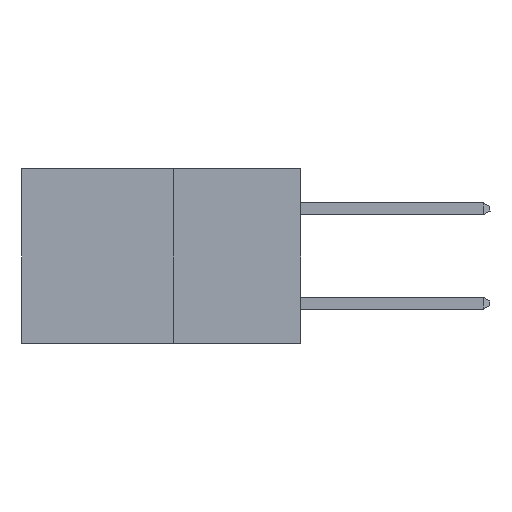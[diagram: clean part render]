
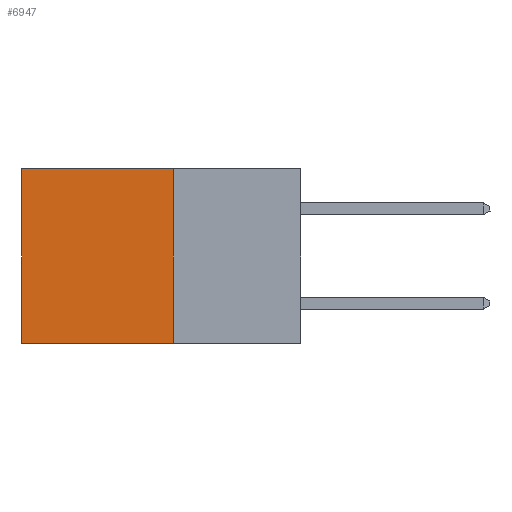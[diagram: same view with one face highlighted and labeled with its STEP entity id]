
A CAD part, left-side view. The second image highlights one B-rep face of the part: STEP entity #6947.
In plain terms, the highlighted planar face has unit normal (-1, 0, 0).
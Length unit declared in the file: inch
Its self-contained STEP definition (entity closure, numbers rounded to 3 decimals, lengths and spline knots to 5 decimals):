
#608 = VERTEX_POINT ( 'NONE', #18790 ) ;
#824 = LINE ( 'NONE', #18918, #17381 ) ;
#1024 = LINE ( 'NONE', #18147, #11940 ) ;
#1056 = CARTESIAN_POINT ( 'NONE',  ( 0.277, 0.27, -0.37 ) ) ;
#1272 = ORIENTED_EDGE ( 'NONE', *, *, #23942, .F. ) ;
#1971 = EDGE_LOOP ( 'NONE', ( #13141, #4662, #1272, #6593 ) ) ;
#3967 = DIRECTION ( 'NONE',  ( 0., 0., -1. ) ) ;
#4662 = ORIENTED_EDGE ( 'NONE', *, *, #21241, .F. ) ;
#6593 = ORIENTED_EDGE ( 'NONE', *, *, #24216, .T. ) ;
#6947 = ADVANCED_FACE ( 'NONE', ( #19543 ), #9834, .F. ) ;
#7674 = VECTOR ( 'NONE', #22424, 39.37008 ) ;
#8910 = AXIS2_PLACEMENT_3D ( 'NONE', #12114, #12168, #12165 ) ;
#9090 = CARTESIAN_POINT ( 'NONE',  ( 0.277, 0.27, 0. ) ) ;
#9834 = PLANE ( 'NONE',  #8910 ) ;
#11188 = CARTESIAN_POINT ( 'NONE',  ( 0.277, 0.59, -0.37 ) ) ;
#11940 = VECTOR ( 'NONE', #20237, 39.37008 ) ;
#12114 = CARTESIAN_POINT ( 'NONE',  ( 0.277, 0.27, -0.37 ) ) ;
#12165 = DIRECTION ( 'NONE',  ( 0., 0., -1. ) ) ;
#12168 = DIRECTION ( 'NONE',  ( 1., 0., 0. ) ) ;
#13141 = ORIENTED_EDGE ( 'NONE', *, *, #23037, .T. ) ;
#13915 = CARTESIAN_POINT ( 'NONE',  ( 0.277, 0.59, 0. ) ) ;
#15247 = CARTESIAN_POINT ( 'NONE',  ( 0.277, 0.27, 0. ) ) ;
#15305 = VERTEX_POINT ( 'NONE', #13915 ) ;
#15718 = LINE ( 'NONE', #9090, #27435 ) ;
#17371 = VERTEX_POINT ( 'NONE', #11188 ) ;
#17381 = VECTOR ( 'NONE', #3967, 39.37008 ) ;
#18147 = CARTESIAN_POINT ( 'NONE',  ( 0.277, 0.59, -0.37 ) ) ;
#18790 = CARTESIAN_POINT ( 'NONE',  ( 0.277, 0.27, -0.37 ) ) ;
#18918 = CARTESIAN_POINT ( 'NONE',  ( 0.277, 0.27, -0.37 ) ) ;
#19543 = FACE_OUTER_BOUND ( 'NONE', #1971, .T. ) ;
#19664 = LINE ( 'NONE', #1056, #7674 ) ;
#20237 = DIRECTION ( 'NONE',  ( 0., 0., -1. ) ) ;
#21241 = EDGE_CURVE ( 'NONE', #608, #17371, #19664, .T. ) ;
#22424 = DIRECTION ( 'NONE',  ( 0., 1., 0. ) ) ;
#23037 = EDGE_CURVE ( 'NONE', #15305, #17371, #1024, .T. ) ;
#23942 = EDGE_CURVE ( 'NONE', #25971, #608, #824, .T. ) ;
#24216 = EDGE_CURVE ( 'NONE', #25971, #15305, #15718, .T. ) ;
#25898 = DIRECTION ( 'NONE',  ( 0., 1., 0. ) ) ;
#25971 = VERTEX_POINT ( 'NONE', #15247 ) ;
#27435 = VECTOR ( 'NONE', #25898, 39.37008 ) ;
